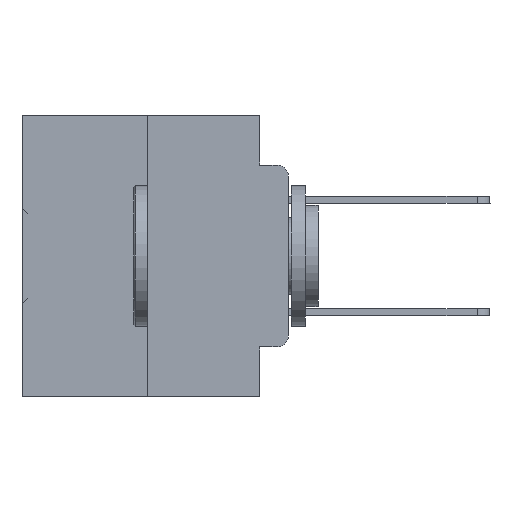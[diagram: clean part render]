
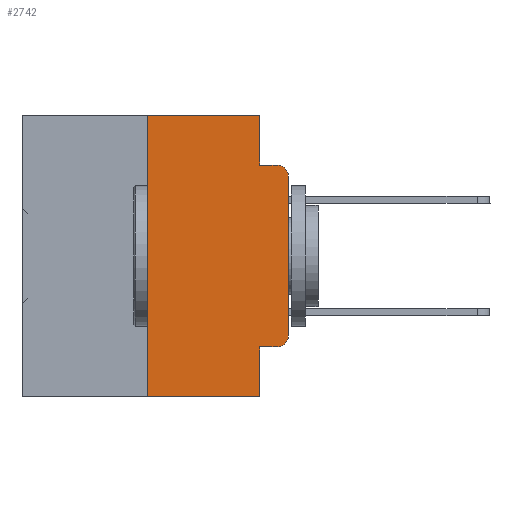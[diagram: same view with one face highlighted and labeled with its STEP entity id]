
A CAD part, left-side view. The second image highlights one B-rep face of the part: STEP entity #2742.
In plain terms, the highlighted planar face has unit normal (-1, 0, 0).
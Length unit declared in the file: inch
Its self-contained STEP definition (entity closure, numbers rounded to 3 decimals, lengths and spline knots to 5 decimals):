
#234 = LINE ( 'NONE', #15983, #12056 ) ;
#520 = EDGE_CURVE ( 'NONE', #14431, #28442, #28699, .T. ) ;
#1621 = VECTOR ( 'NONE', #19604, 39.37008 ) ;
#1709 = ORIENTED_EDGE ( 'NONE', *, *, #31085, .F. ) ;
#2742 = ADVANCED_FACE ( 'NONE', ( #29092 ), #8505, .F. ) ;
#3146 = DIRECTION ( 'NONE',  ( 0., 0., -1. ) ) ;
#4639 = EDGE_CURVE ( 'NONE', #27657, #32226, #33682, .T. ) ;
#5929 = CARTESIAN_POINT ( 'NONE',  ( 0., 0., 0. ) ) ;
#6670 = DIRECTION ( 'NONE',  ( 0., -1., 0. ) ) ;
#6829 = AXIS2_PLACEMENT_3D ( 'NONE', #10129, #21940, #27815 ) ;
#7643 = ORIENTED_EDGE ( 'NONE', *, *, #30910, .F. ) ;
#7896 = CARTESIAN_POINT ( 'NONE',  ( 0., 0.051, 0. ) ) ;
#7918 = CARTESIAN_POINT ( 'NONE',  ( 0., 0., -0.3915 ) ) ;
#8458 = CIRCLE ( 'NONE', #6829, 0.02 ) ;
#8505 = PLANE ( 'NONE',  #31032 ) ;
#9202 = CARTESIAN_POINT ( 'NONE',  ( 0., 0.02, -0.0885 ) ) ;
#9886 = VECTOR ( 'NONE', #28776, 39.37008 ) ;
#9946 = DIRECTION ( 'NONE',  ( 0., -1., 0. ) ) ;
#10129 = CARTESIAN_POINT ( 'NONE',  ( 0., 0.02, -0.3915 ) ) ;
#10888 = CARTESIAN_POINT ( 'NONE',  ( 0., 0.051, -0.4115 ) ) ;
#11310 = DIRECTION ( 'NONE',  ( 0., 0., -1. ) ) ;
#11701 = VECTOR ( 'NONE', #14675, 39.37008 ) ;
#12044 = DIRECTION ( 'NONE',  ( -1., 0., 0. ) ) ;
#12056 = VECTOR ( 'NONE', #33406, 39.37008 ) ;
#12543 = DIRECTION ( 'NONE',  ( 0., 0., -1. ) ) ;
#13213 = DIRECTION ( 'NONE',  ( 0., -1., 0. ) ) ;
#13308 = VERTEX_POINT ( 'NONE', #29392 ) ;
#13792 = VERTEX_POINT ( 'NONE', #22473 ) ;
#14191 = CARTESIAN_POINT ( 'NONE',  ( 0., 0.25, 0. ) ) ;
#14340 = CARTESIAN_POINT ( 'NONE',  ( 0., 0.051, 0. ) ) ;
#14431 = VERTEX_POINT ( 'NONE', #10888 ) ;
#14675 = DIRECTION ( 'NONE',  ( 0., 0., 1. ) ) ;
#15983 = CARTESIAN_POINT ( 'NONE',  ( 0., 0.25, 0. ) ) ;
#17273 = CARTESIAN_POINT ( 'NONE',  ( 0., 0.051, 0. ) ) ;
#18828 = CARTESIAN_POINT ( 'NONE',  ( 0., 0.25, -0.5 ) ) ;
#19604 = DIRECTION ( 'NONE',  ( 0., 0., -1. ) ) ;
#19614 = VERTEX_POINT ( 'NONE', #9202 ) ;
#20557 = VECTOR ( 'NONE', #6670, 39.37008 ) ;
#20786 = LINE ( 'NONE', #32951, #27625 ) ;
#20942 = VECTOR ( 'NONE', #13213, 39.37008 ) ;
#21161 = ORIENTED_EDGE ( 'NONE', *, *, #520, .T. ) ;
#21410 = CARTESIAN_POINT ( 'NONE',  ( 0., 0.051, -0.0885 ) ) ;
#21465 = ORIENTED_EDGE ( 'NONE', *, *, #35937, .T. ) ;
#21645 = CARTESIAN_POINT ( 'NONE',  ( 0., 0.051, -0.0885 ) ) ;
#21940 = DIRECTION ( 'NONE',  ( -1., 0., 0. ) ) ;
#22417 = EDGE_LOOP ( 'NONE', ( #21465, #22810, #36920, #37102, #7643, #33547, #22578, #1709, #21161, #31837 ) ) ;
#22473 = CARTESIAN_POINT ( 'NONE',  ( 0., 0.051, -0.5 ) ) ;
#22578 = ORIENTED_EDGE ( 'NONE', *, *, #36459, .T. ) ;
#22810 = ORIENTED_EDGE ( 'NONE', *, *, #28189, .T. ) ;
#22944 = EDGE_CURVE ( 'NONE', #28442, #29032, #8458, .T. ) ;
#26033 = AXIS2_PLACEMENT_3D ( 'NONE', #29624, #12044, #3146 ) ;
#27625 = VECTOR ( 'NONE', #9946, 39.37008 ) ;
#27657 = VERTEX_POINT ( 'NONE', #17273 ) ;
#27815 = DIRECTION ( 'NONE',  ( 0., 0., -1. ) ) ;
#28189 = EDGE_CURVE ( 'NONE', #13308, #19614, #30824, .T. ) ;
#28442 = VERTEX_POINT ( 'NONE', #33909 ) ;
#28556 = VERTEX_POINT ( 'NONE', #14191 ) ;
#28699 = LINE ( 'NONE', #30864, #20942 ) ;
#28776 = DIRECTION ( 'NONE',  ( 0., -1., 0. ) ) ;
#28855 = DIRECTION ( 'NONE',  ( 1., 0., 0. ) ) ;
#29009 = LINE ( 'NONE', #5929, #11701 ) ;
#29032 = VERTEX_POINT ( 'NONE', #7918 ) ;
#29092 = FACE_OUTER_BOUND ( 'NONE', #22417, .T. ) ;
#29392 = CARTESIAN_POINT ( 'NONE',  ( 0., 0., -0.1085 ) ) ;
#29453 = LINE ( 'NONE', #7896, #1621 ) ;
#29624 = CARTESIAN_POINT ( 'NONE',  ( 0., 0.02, -0.1085 ) ) ;
#30824 = CIRCLE ( 'NONE', #26033, 0.02 ) ;
#30864 = CARTESIAN_POINT ( 'NONE',  ( 0., 0.051, -0.4115 ) ) ;
#30910 = EDGE_CURVE ( 'NONE', #28556, #27657, #20786, .T. ) ;
#30939 = VERTEX_POINT ( 'NONE', #18828 ) ;
#31032 = AXIS2_PLACEMENT_3D ( 'NONE', #35070, #28855, #12543 ) ;
#31085 = EDGE_CURVE ( 'NONE', #14431, #13792, #29453, .T. ) ;
#31576 = EDGE_CURVE ( 'NONE', #30939, #28556, #234, .T. ) ;
#31837 = ORIENTED_EDGE ( 'NONE', *, *, #22944, .T. ) ;
#31921 = CARTESIAN_POINT ( 'NONE',  ( 0., 0.473, -0.5 ) ) ;
#32158 = LINE ( 'NONE', #31921, #9886 ) ;
#32165 = EDGE_CURVE ( 'NONE', #32226, #19614, #34689, .T. ) ;
#32226 = VERTEX_POINT ( 'NONE', #21645 ) ;
#32951 = CARTESIAN_POINT ( 'NONE',  ( 0., 0.473, 0. ) ) ;
#33406 = DIRECTION ( 'NONE',  ( 0., 0., 1. ) ) ;
#33547 = ORIENTED_EDGE ( 'NONE', *, *, #31576, .F. ) ;
#33682 = LINE ( 'NONE', #14340, #35488 ) ;
#33909 = CARTESIAN_POINT ( 'NONE',  ( 0., 0.02, -0.4115 ) ) ;
#34689 = LINE ( 'NONE', #21410, #20557 ) ;
#35070 = CARTESIAN_POINT ( 'NONE',  ( 0., 0.473, 0. ) ) ;
#35488 = VECTOR ( 'NONE', #11310, 39.37008 ) ;
#35937 = EDGE_CURVE ( 'NONE', #29032, #13308, #29009, .T. ) ;
#36459 = EDGE_CURVE ( 'NONE', #30939, #13792, #32158, .T. ) ;
#36920 = ORIENTED_EDGE ( 'NONE', *, *, #32165, .F. ) ;
#37102 = ORIENTED_EDGE ( 'NONE', *, *, #4639, .F. ) ;
